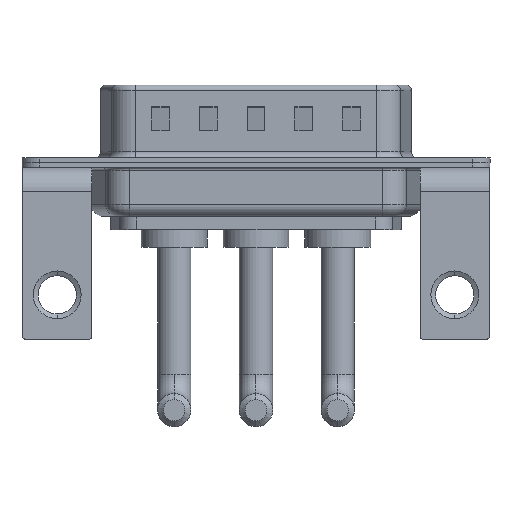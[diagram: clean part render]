
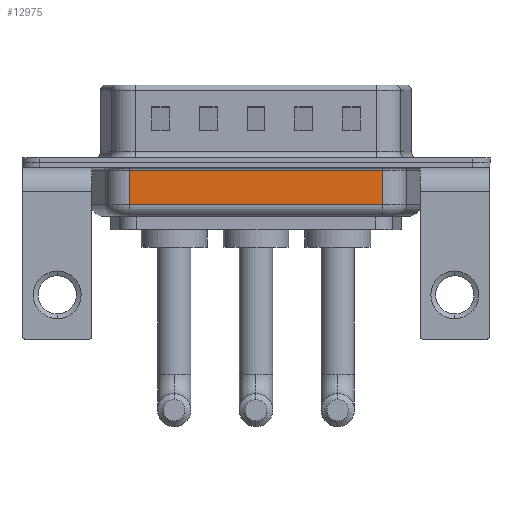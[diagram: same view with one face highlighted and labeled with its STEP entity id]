
A CAD part, front view. The second image highlights one B-rep face of the part: STEP entity #12975.
In plain terms, the highlighted planar face has unit normal (0, -1, 0).
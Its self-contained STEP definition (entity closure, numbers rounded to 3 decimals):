
#612 = LINE ( 'NONE', #9506, #2129 ) ;
#764 = VERTEX_POINT ( 'NONE', #4989 ) ;
#1512 = CARTESIAN_POINT ( 'NONE',  ( 6.031, -5.35, -0.65 ) ) ;
#1543 = LINE ( 'NONE', #15198, #9333 ) ;
#1698 = DIRECTION ( 'NONE',  ( 1., 0., 0. ) ) ;
#2080 = DIRECTION ( 'NONE',  ( 0., 1., 0. ) ) ;
#2129 = VECTOR ( 'NONE', #6927, 1000. ) ;
#2521 = EDGE_CURVE ( 'NONE', #5444, #4355, #612, .T. ) ;
#2605 = ORIENTED_EDGE ( 'NONE', *, *, #9691, .T. ) ;
#2909 = EDGE_LOOP ( 'NONE', ( #6653, #14996, #2605, #15545 ) ) ;
#3413 = CARTESIAN_POINT ( 'NONE',  ( 6.031, -5.35, -4.5 ) ) ;
#3751 = CARTESIAN_POINT ( 'NONE',  ( 27.269, -5.35, -3.5 ) ) ;
#4355 = VERTEX_POINT ( 'NONE', #1512 ) ;
#4664 = DIRECTION ( 'NONE',  ( 0., 0., 1. ) ) ;
#4989 = CARTESIAN_POINT ( 'NONE',  ( 6.031, -5.35, -3.5 ) ) ;
#5122 = EDGE_CURVE ( 'NONE', #764, #4355, #1543, .T. ) ;
#5444 = VERTEX_POINT ( 'NONE', #8867 ) ;
#5928 = VERTEX_POINT ( 'NONE', #3751 ) ;
#6621 = DIRECTION ( 'NONE',  ( 0., 0., 1. ) ) ;
#6653 = ORIENTED_EDGE ( 'NONE', *, *, #5122, .F. ) ;
#6821 = AXIS2_PLACEMENT_3D ( 'NONE', #3413, #2080, #4664 ) ;
#6927 = DIRECTION ( 'NONE',  ( -1., 0., 0. ) ) ;
#7797 = DIRECTION ( 'NONE',  ( 0., 0., 1. ) ) ;
#8867 = CARTESIAN_POINT ( 'NONE',  ( 27.269, -5.35, -0.65 ) ) ;
#9211 = LINE ( 'NONE', #10290, #9401 ) ;
#9333 = VECTOR ( 'NONE', #7797, 1000. ) ;
#9401 = VECTOR ( 'NONE', #6621, 1000. ) ;
#9506 = CARTESIAN_POINT ( 'NONE',  ( 6.031, -5.35, -0.65 ) ) ;
#9691 = EDGE_CURVE ( 'NONE', #5928, #5444, #9211, .T. ) ;
#9796 = PLANE ( 'NONE',  #6821 ) ;
#10290 = CARTESIAN_POINT ( 'NONE',  ( 27.269, -5.35, -4.5 ) ) ;
#10424 = LINE ( 'NONE', #10509, #15722 ) ;
#10509 = CARTESIAN_POINT ( 'NONE',  ( 6.031, -5.35, -3.5 ) ) ;
#12975 = ADVANCED_FACE ( 'NONE', ( #13479 ), #9796, .F. ) ;
#13479 = FACE_OUTER_BOUND ( 'NONE', #2909, .T. ) ;
#14996 = ORIENTED_EDGE ( 'NONE', *, *, #15474, .T. ) ;
#15198 = CARTESIAN_POINT ( 'NONE',  ( 6.031, -5.35, -4.5 ) ) ;
#15474 = EDGE_CURVE ( 'NONE', #764, #5928, #10424, .T. ) ;
#15545 = ORIENTED_EDGE ( 'NONE', *, *, #2521, .T. ) ;
#15722 = VECTOR ( 'NONE', #1698, 1000. ) ;
